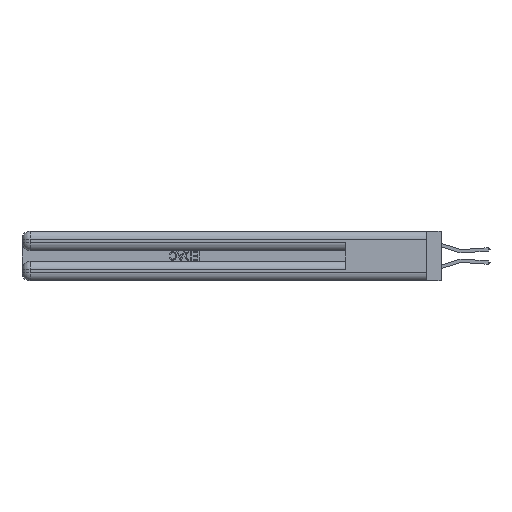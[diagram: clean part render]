
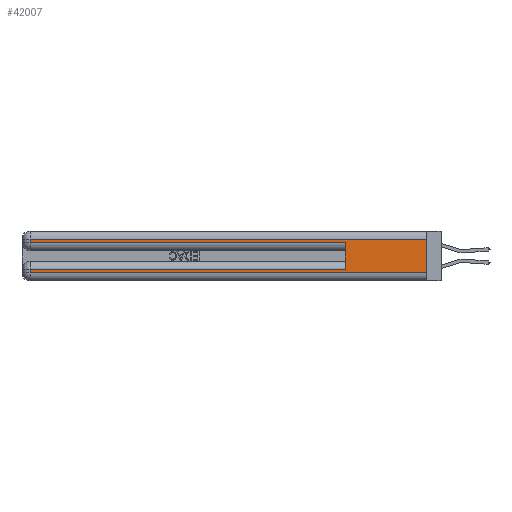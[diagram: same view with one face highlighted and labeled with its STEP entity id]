
A CAD part, left-side view. The second image highlights one B-rep face of the part: STEP entity #42007.
In plain terms, the highlighted planar face has unit normal (-1, 0, 0).
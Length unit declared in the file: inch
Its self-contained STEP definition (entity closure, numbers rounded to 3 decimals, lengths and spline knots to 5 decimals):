
#632 = VERTEX_POINT ( 'NONE', #16585 ) ;
#1363 = CARTESIAN_POINT ( 'NONE',  ( 0., 0., 0.06 ) ) ;
#1661 = CARTESIAN_POINT ( 'NONE',  ( 0., 0., 0.31 ) ) ;
#3549 = DIRECTION ( 'NONE',  ( 1., 0., 0. ) ) ;
#3746 = VERTEX_POINT ( 'NONE', #9335 ) ;
#4021 = DIRECTION ( 'NONE',  ( 0., 0., -1. ) ) ;
#4397 = LINE ( 'NONE', #24748, #24691 ) ;
#7823 = ORIENTED_EDGE ( 'NONE', *, *, #14020, .F. ) ;
#7928 = CARTESIAN_POINT ( 'NONE',  ( 0., 2.94, 0.31 ) ) ;
#8354 = VECTOR ( 'NONE', #8544, 39.37008 ) ;
#8544 = DIRECTION ( 'NONE',  ( 0., 1., 0. ) ) ;
#8994 = LINE ( 'NONE', #34658, #8354 ) ;
#9335 = CARTESIAN_POINT ( 'NONE',  ( 0., 2.94, 0.06 ) ) ;
#9932 = PLANE ( 'NONE',  #26818 ) ;
#10095 = DIRECTION ( 'NONE',  ( 0., 0., 1. ) ) ;
#10323 = VERTEX_POINT ( 'NONE', #1363 ) ;
#11000 = DIRECTION ( 'NONE',  ( 0., 0., -1. ) ) ;
#11893 = CARTESIAN_POINT ( 'NONE',  ( 0., 2.94, 0.285 ) ) ;
#13525 = VERTEX_POINT ( 'NONE', #26346 ) ;
#13643 = LINE ( 'NONE', #19652, #15399 ) ;
#14020 = EDGE_CURVE ( 'NONE', #632, #13525, #40520, .T. ) ;
#14357 = EDGE_LOOP ( 'NONE', ( #31278, #37604, #25331, #22284, #7823, #14656, #45654, #29016 ) ) ;
#14601 = EDGE_CURVE ( 'NONE', #47325, #13525, #41047, .T. ) ;
#14656 = ORIENTED_EDGE ( 'NONE', *, *, #48811, .T. ) ;
#15399 = VECTOR ( 'NONE', #34971, 39.37008 ) ;
#16585 = CARTESIAN_POINT ( 'NONE',  ( 0., 0.6, 0.085 ) ) ;
#16717 = CARTESIAN_POINT ( 'NONE',  ( 0., 0., 0.285 ) ) ;
#16780 = CARTESIAN_POINT ( 'NONE',  ( 0., 0., 0.31 ) ) ;
#18186 = EDGE_CURVE ( 'NONE', #3746, #10323, #4397, .T. ) ;
#18426 = CARTESIAN_POINT ( 'NONE',  ( 0., 0., 0.37 ) ) ;
#19195 = CARTESIAN_POINT ( 'NONE',  ( 0., 2.94, 0.37 ) ) ;
#19652 = CARTESIAN_POINT ( 'NONE',  ( 0., 0., 0.37 ) ) ;
#20271 = VECTOR ( 'NONE', #10095, 39.37008 ) ;
#20427 = LINE ( 'NONE', #19195, #40057 ) ;
#21346 = VERTEX_POINT ( 'NONE', #16780 ) ;
#21582 = LINE ( 'NONE', #1661, #29334 ) ;
#22284 = ORIENTED_EDGE ( 'NONE', *, *, #14601, .T. ) ;
#24691 = VECTOR ( 'NONE', #31725, 39.37008 ) ;
#24748 = CARTESIAN_POINT ( 'NONE',  ( 0., 0., 0.06 ) ) ;
#25331 = ORIENTED_EDGE ( 'NONE', *, *, #47427, .T. ) ;
#25974 = EDGE_CURVE ( 'NONE', #21346, #36410, #21582, .T. ) ;
#26346 = CARTESIAN_POINT ( 'NONE',  ( 0., 0.6, 0.285 ) ) ;
#26818 = AXIS2_PLACEMENT_3D ( 'NONE', #18426, #3549, #45130 ) ;
#28352 = DIRECTION ( 'NONE',  ( 0., 1., 0. ) ) ;
#28779 = FACE_OUTER_BOUND ( 'NONE', #14357, .T. ) ;
#28916 = EDGE_CURVE ( 'NONE', #30915, #3746, #29326, .T. ) ;
#29016 = ORIENTED_EDGE ( 'NONE', *, *, #18186, .T. ) ;
#29105 = CARTESIAN_POINT ( 'NONE',  ( 0., 0.6, 0.145 ) ) ;
#29326 = LINE ( 'NONE', #49387, #31064 ) ;
#29334 = VECTOR ( 'NONE', #28352, 39.37008 ) ;
#30565 = EDGE_CURVE ( 'NONE', #21346, #10323, #13643, .T. ) ;
#30915 = VERTEX_POINT ( 'NONE', #33898 ) ;
#31064 = VECTOR ( 'NONE', #11000, 39.37008 ) ;
#31278 = ORIENTED_EDGE ( 'NONE', *, *, #30565, .F. ) ;
#31725 = DIRECTION ( 'NONE',  ( 0., -1., 0. ) ) ;
#33898 = CARTESIAN_POINT ( 'NONE',  ( 0., 2.94, 0.085 ) ) ;
#34658 = CARTESIAN_POINT ( 'NONE',  ( 0., 0., 0.085 ) ) ;
#34971 = DIRECTION ( 'NONE',  ( 0., 0., -1. ) ) ;
#35713 = VECTOR ( 'NONE', #43864, 39.37008 ) ;
#36410 = VERTEX_POINT ( 'NONE', #7928 ) ;
#37604 = ORIENTED_EDGE ( 'NONE', *, *, #25974, .T. ) ;
#40057 = VECTOR ( 'NONE', #4021, 39.37008 ) ;
#40520 = LINE ( 'NONE', #29105, #20271 ) ;
#41047 = LINE ( 'NONE', #16717, #35713 ) ;
#42007 = ADVANCED_FACE ( 'NONE', ( #28779 ), #9932, .F. ) ;
#43864 = DIRECTION ( 'NONE',  ( 0., -1., 0. ) ) ;
#45130 = DIRECTION ( 'NONE',  ( 0., 0., -1. ) ) ;
#45654 = ORIENTED_EDGE ( 'NONE', *, *, #28916, .T. ) ;
#47325 = VERTEX_POINT ( 'NONE', #11893 ) ;
#47427 = EDGE_CURVE ( 'NONE', #36410, #47325, #20427, .T. ) ;
#48811 = EDGE_CURVE ( 'NONE', #632, #30915, #8994, .T. ) ;
#49387 = CARTESIAN_POINT ( 'NONE',  ( 0., 2.94, 0.37 ) ) ;
